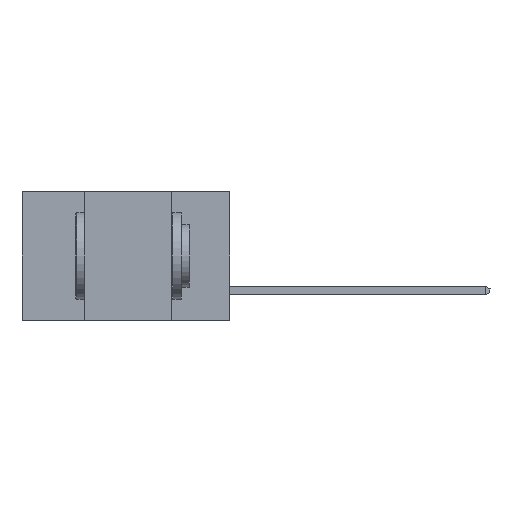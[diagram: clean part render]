
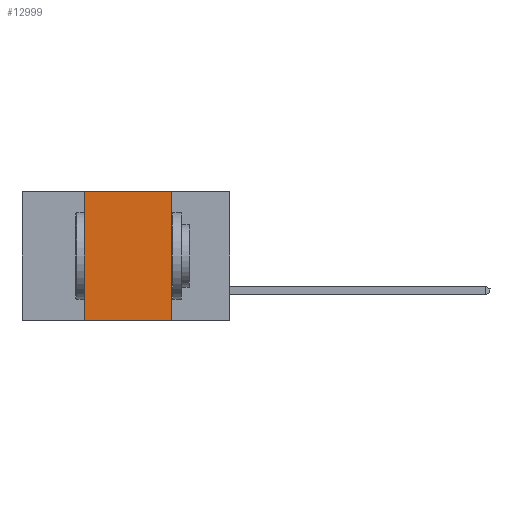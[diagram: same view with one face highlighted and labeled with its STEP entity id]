
A CAD part, left-side view. The second image highlights one B-rep face of the part: STEP entity #12999.
In plain terms, the highlighted planar face has unit normal (-1, 0, 0).
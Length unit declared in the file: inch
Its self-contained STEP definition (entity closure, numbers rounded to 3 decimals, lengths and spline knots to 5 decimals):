
#57 = LINE ( 'NONE', #5023, #15337 ) ;
#1220 = VERTEX_POINT ( 'NONE', #8575 ) ;
#1813 = CARTESIAN_POINT ( 'NONE',  ( 0., 0.6, 0. ) ) ;
#1910 = AXIS2_PLACEMENT_3D ( 'NONE', #13107, #11887, #7217 ) ;
#2885 = VERTEX_POINT ( 'NONE', #3512 ) ;
#3497 = EDGE_CURVE ( 'NONE', #10062, #2885, #4240, .T. ) ;
#3512 = CARTESIAN_POINT ( 'NONE',  ( 0., 0.17, 0. ) ) ;
#4069 = VECTOR ( 'NONE', #12625, 39.37008 ) ;
#4111 = CARTESIAN_POINT ( 'NONE',  ( 0., 0.6, -0.37 ) ) ;
#4240 = LINE ( 'NONE', #1813, #5798 ) ;
#4501 = LINE ( 'NONE', #10760, #11675 ) ;
#4876 = ORIENTED_EDGE ( 'NONE', *, *, #15167, .F. ) ;
#5023 = CARTESIAN_POINT ( 'NONE',  ( 0., 0.42, -0.37 ) ) ;
#5798 = VECTOR ( 'NONE', #14209, 39.37008 ) ;
#7058 = ORIENTED_EDGE ( 'NONE', *, *, #7970, .T. ) ;
#7119 = ORIENTED_EDGE ( 'NONE', *, *, #11671, .F. ) ;
#7217 = DIRECTION ( 'NONE',  ( 0., 0., -1. ) ) ;
#7970 = EDGE_CURVE ( 'NONE', #1220, #9761, #11256, .T. ) ;
#8197 = PLANE ( 'NONE',  #1910 ) ;
#8431 = FACE_OUTER_BOUND ( 'NONE', #13989, .T. ) ;
#8575 = CARTESIAN_POINT ( 'NONE',  ( 0., 0.42, -0.37 ) ) ;
#9761 = VERTEX_POINT ( 'NONE', #14878 ) ;
#10062 = VERTEX_POINT ( 'NONE', #12520 ) ;
#10760 = CARTESIAN_POINT ( 'NONE',  ( 0., 0.17, -0.37 ) ) ;
#11041 = DIRECTION ( 'NONE',  ( 0., 0., 1. ) ) ;
#11256 = LINE ( 'NONE', #4111, #4069 ) ;
#11671 = EDGE_CURVE ( 'NONE', #2885, #9761, #4501, .T. ) ;
#11675 = VECTOR ( 'NONE', #13270, 39.37008 ) ;
#11870 = ORIENTED_EDGE ( 'NONE', *, *, #3497, .F. ) ;
#11887 = DIRECTION ( 'NONE',  ( 1., 0., 0. ) ) ;
#12520 = CARTESIAN_POINT ( 'NONE',  ( 0., 0.42, 0. ) ) ;
#12625 = DIRECTION ( 'NONE',  ( 0., -1., 0. ) ) ;
#12999 = ADVANCED_FACE ( 'NONE', ( #8431 ), #8197, .F. ) ;
#13107 = CARTESIAN_POINT ( 'NONE',  ( 0., 0.6, 0. ) ) ;
#13270 = DIRECTION ( 'NONE',  ( 0., 0., -1. ) ) ;
#13989 = EDGE_LOOP ( 'NONE', ( #7119, #11870, #4876, #7058 ) ) ;
#14209 = DIRECTION ( 'NONE',  ( 0., -1., 0. ) ) ;
#14878 = CARTESIAN_POINT ( 'NONE',  ( 0., 0.17, -0.37 ) ) ;
#15167 = EDGE_CURVE ( 'NONE', #1220, #10062, #57, .T. ) ;
#15337 = VECTOR ( 'NONE', #11041, 39.37008 ) ;
